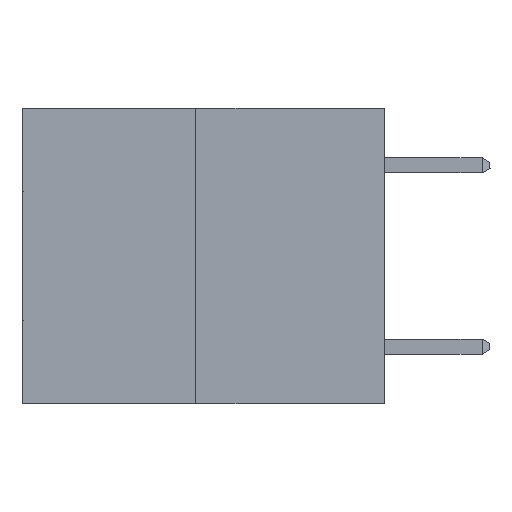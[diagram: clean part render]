
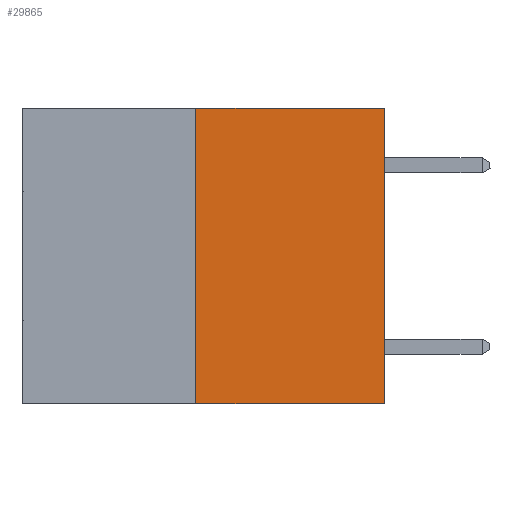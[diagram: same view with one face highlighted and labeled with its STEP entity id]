
A CAD part, left-side view. The second image highlights one B-rep face of the part: STEP entity #29865.
In plain terms, the highlighted planar face has unit normal (-1, 0, 0).
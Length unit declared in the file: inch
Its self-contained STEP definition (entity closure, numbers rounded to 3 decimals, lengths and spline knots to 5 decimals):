
#312 = VECTOR ( 'NONE', #19488, 39.37008 ) ;
#2071 = CARTESIAN_POINT ( 'NONE',  ( 0., 0.6, 0. ) ) ;
#4118 = FACE_OUTER_BOUND ( 'NONE', #16284, .T. ) ;
#6211 = CARTESIAN_POINT ( 'NONE',  ( 0., 0.312, 0. ) ) ;
#6261 = EDGE_CURVE ( 'NONE', #31723, #17496, #7139, .T. ) ;
#7019 = CARTESIAN_POINT ( 'NONE',  ( 0., 0.6, 0. ) ) ;
#7139 = LINE ( 'NONE', #31319, #31328 ) ;
#8997 = DIRECTION ( 'NONE',  ( 0., -1., 0. ) ) ;
#9641 = DIRECTION ( 'NONE',  ( 0., 0., 1. ) ) ;
#10301 = VERTEX_POINT ( 'NONE', #24648 ) ;
#11510 = VECTOR ( 'NONE', #9641, 39.37008 ) ;
#12517 = ORIENTED_EDGE ( 'NONE', *, *, #19953, .T. ) ;
#13931 = ORIENTED_EDGE ( 'NONE', *, *, #6261, .F. ) ;
#14368 = LINE ( 'NONE', #7019, #312 ) ;
#14461 = DIRECTION ( 'NONE',  ( 1., 0., 0. ) ) ;
#14679 = PLANE ( 'NONE',  #19164 ) ;
#14907 = LINE ( 'NONE', #31168, #18811 ) ;
#15273 = CARTESIAN_POINT ( 'NONE',  ( 0., 0., 0. ) ) ;
#15422 = LINE ( 'NONE', #16935, #11510 ) ;
#15585 = ORIENTED_EDGE ( 'NONE', *, *, #21529, .F. ) ;
#16284 = EDGE_LOOP ( 'NONE', ( #13931, #26452, #12517, #15585 ) ) ;
#16935 = CARTESIAN_POINT ( 'NONE',  ( 0., 0., 0. ) ) ;
#17496 = VERTEX_POINT ( 'NONE', #6211 ) ;
#18811 = VECTOR ( 'NONE', #8997, 39.37008 ) ;
#19164 = AXIS2_PLACEMENT_3D ( 'NONE', #2071, #14461, #27228 ) ;
#19488 = DIRECTION ( 'NONE',  ( 0., -1., 0. ) ) ;
#19953 = EDGE_CURVE ( 'NONE', #10301, #29422, #15422, .T. ) ;
#21529 = EDGE_CURVE ( 'NONE', #17496, #29422, #14368, .T. ) ;
#23182 = CARTESIAN_POINT ( 'NONE',  ( 0., 0.312, -0.49 ) ) ;
#23528 = DIRECTION ( 'NONE',  ( 0., 0., 1. ) ) ;
#24648 = CARTESIAN_POINT ( 'NONE',  ( 0., 0., -0.49 ) ) ;
#24995 = EDGE_CURVE ( 'NONE', #31723, #10301, #14907, .T. ) ;
#26452 = ORIENTED_EDGE ( 'NONE', *, *, #24995, .T. ) ;
#27228 = DIRECTION ( 'NONE',  ( 0., 0., -1. ) ) ;
#29422 = VERTEX_POINT ( 'NONE', #15273 ) ;
#29865 = ADVANCED_FACE ( 'NONE', ( #4118 ), #14679, .F. ) ;
#31168 = CARTESIAN_POINT ( 'NONE',  ( 0., 0.6, -0.49 ) ) ;
#31319 = CARTESIAN_POINT ( 'NONE',  ( 0., 0.312, -0.49 ) ) ;
#31328 = VECTOR ( 'NONE', #23528, 39.37008 ) ;
#31723 = VERTEX_POINT ( 'NONE', #23182 ) ;
